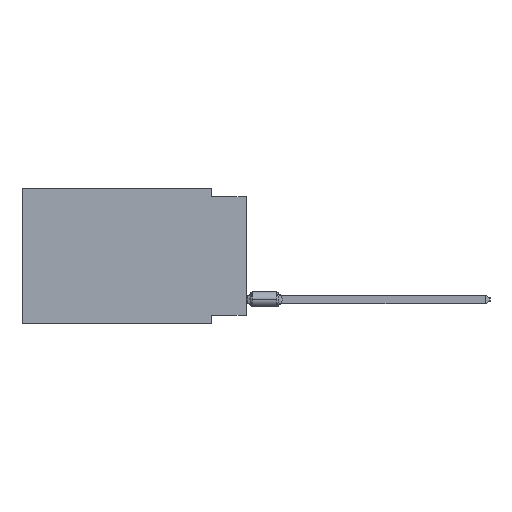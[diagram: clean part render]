
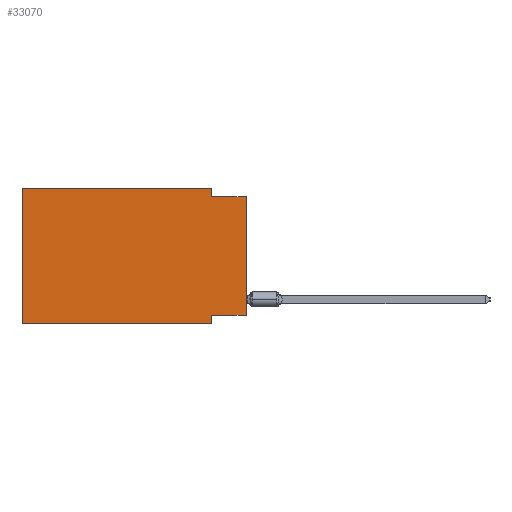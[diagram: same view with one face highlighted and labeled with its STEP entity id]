
A CAD part, left-side view. The second image highlights one B-rep face of the part: STEP entity #33070.
In plain terms, the highlighted planar face has unit normal (-1, 0, 0).
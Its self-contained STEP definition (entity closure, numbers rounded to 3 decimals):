
#898 = VERTEX_POINT ( 'NONE', #55779 ) ;
#2463 = VECTOR ( 'NONE', #65343, 1000. ) ;
#4988 = CARTESIAN_POINT ( 'NONE',  ( 0., 0., -9.271 ) ) ;
#7113 = CARTESIAN_POINT ( 'NONE',  ( 0., 16.383, 0. ) ) ;
#7349 = DIRECTION ( 'NONE',  ( 0., 0., -1. ) ) ;
#8289 = LINE ( 'NONE', #16024, #42178 ) ;
#9789 = VECTOR ( 'NONE', #66621, 1000. ) ;
#11398 = CARTESIAN_POINT ( 'NONE',  ( 0., 16.383, 0. ) ) ;
#13105 = CARTESIAN_POINT ( 'NONE',  ( 0., 0., -0.635 ) ) ;
#13877 = CARTESIAN_POINT ( 'NONE',  ( 0., 16.383, 0. ) ) ;
#13968 = LINE ( 'NONE', #78731, #74807 ) ;
#14330 = DIRECTION ( 'NONE',  ( 0., 1., 0. ) ) ;
#14442 = DIRECTION ( 'NONE',  ( 0., -1., 0. ) ) ;
#16024 = CARTESIAN_POINT ( 'NONE',  ( 0., 0., -9.271 ) ) ;
#18161 = CARTESIAN_POINT ( 'NONE',  ( 0., 0., -0.635 ) ) ;
#18649 = CARTESIAN_POINT ( 'NONE',  ( 0., 2.54, -9.906 ) ) ;
#18819 = EDGE_LOOP ( 'NONE', ( #31350, #49505, #48549, #21379, #64350, #65638, #46109, #35503 ) ) ;
#19003 = DIRECTION ( 'NONE',  ( 1., 0., 0. ) ) ;
#20897 = LINE ( 'NONE', #7113, #51537 ) ;
#21379 = ORIENTED_EDGE ( 'NONE', *, *, #43178, .F. ) ;
#22263 = EDGE_CURVE ( 'NONE', #898, #44504, #66472, .T. ) ;
#25463 = FACE_OUTER_BOUND ( 'NONE', #18819, .T. ) ;
#26371 = EDGE_CURVE ( 'NONE', #33821, #83143, #81209, .T. ) ;
#29829 = DIRECTION ( 'NONE',  ( 0., 0., 1. ) ) ;
#31350 = ORIENTED_EDGE ( 'NONE', *, *, #26371, .T. ) ;
#33070 = ADVANCED_FACE ( 'NONE', ( #25463 ), #58725, .F. ) ;
#33551 = VECTOR ( 'NONE', #66620, 1000. ) ;
#33821 = VERTEX_POINT ( 'NONE', #4988 ) ;
#34724 = AXIS2_PLACEMENT_3D ( 'NONE', #51799, #19003, #45318 ) ;
#35503 = ORIENTED_EDGE ( 'NONE', *, *, #42030, .F. ) ;
#39844 = LINE ( 'NONE', #40260, #33551 ) ;
#40260 = CARTESIAN_POINT ( 'NONE',  ( 0., 16.383, -9.906 ) ) ;
#42030 = EDGE_CURVE ( 'NONE', #33821, #898, #8289, .T. ) ;
#42178 = VECTOR ( 'NONE', #14330, 1000. ) ;
#43178 = EDGE_CURVE ( 'NONE', #59850, #58900, #20897, .T. ) ;
#44185 = LINE ( 'NONE', #11398, #2463 ) ;
#44504 = VERTEX_POINT ( 'NONE', #18649 ) ;
#44828 = CARTESIAN_POINT ( 'NONE',  ( 0., 2.54, 0. ) ) ;
#45318 = DIRECTION ( 'NONE',  ( 0., 0., -1. ) ) ;
#46109 = ORIENTED_EDGE ( 'NONE', *, *, #22263, .F. ) ;
#48549 = ORIENTED_EDGE ( 'NONE', *, *, #66358, .F. ) ;
#49505 = ORIENTED_EDGE ( 'NONE', *, *, #58242, .F. ) ;
#49683 = VERTEX_POINT ( 'NONE', #84803 ) ;
#51537 = VECTOR ( 'NONE', #14442, 1000. ) ;
#51799 = CARTESIAN_POINT ( 'NONE',  ( 0., 16.383, 0. ) ) ;
#53158 = EDGE_CURVE ( 'NONE', #58434, #59850, #44185, .T. ) ;
#54459 = CARTESIAN_POINT ( 'NONE',  ( 0., 0., 0. ) ) ;
#55779 = CARTESIAN_POINT ( 'NONE',  ( 0., 2.54, -9.271 ) ) ;
#58242 = EDGE_CURVE ( 'NONE', #49683, #83143, #59727, .T. ) ;
#58434 = VERTEX_POINT ( 'NONE', #71283 ) ;
#58725 = PLANE ( 'NONE',  #34724 ) ;
#58900 = VERTEX_POINT ( 'NONE', #44828 ) ;
#59727 = LINE ( 'NONE', #13105, #9789 ) ;
#59850 = VERTEX_POINT ( 'NONE', #13877 ) ;
#64350 = ORIENTED_EDGE ( 'NONE', *, *, #53158, .F. ) ;
#65343 = DIRECTION ( 'NONE',  ( 0., 0., 1. ) ) ;
#65638 = ORIENTED_EDGE ( 'NONE', *, *, #69111, .T. ) ;
#66209 = DIRECTION ( 'NONE',  ( 0., 0., -1. ) ) ;
#66358 = EDGE_CURVE ( 'NONE', #58900, #49683, #13968, .T. ) ;
#66472 = LINE ( 'NONE', #77714, #70105 ) ;
#66620 = DIRECTION ( 'NONE',  ( 0., -1., 0. ) ) ;
#66621 = DIRECTION ( 'NONE',  ( 0., -1., 0. ) ) ;
#69111 = EDGE_CURVE ( 'NONE', #58434, #44504, #39844, .T. ) ;
#70105 = VECTOR ( 'NONE', #7349, 1000. ) ;
#71283 = CARTESIAN_POINT ( 'NONE',  ( 0., 16.383, -9.906 ) ) ;
#74807 = VECTOR ( 'NONE', #66209, 1000. ) ;
#77714 = CARTESIAN_POINT ( 'NONE',  ( 0., 2.54, -9.906 ) ) ;
#78093 = VECTOR ( 'NONE', #29829, 1000. ) ;
#78731 = CARTESIAN_POINT ( 'NONE',  ( 0., 2.54, 0. ) ) ;
#81209 = LINE ( 'NONE', #54459, #78093 ) ;
#83143 = VERTEX_POINT ( 'NONE', #18161 ) ;
#84803 = CARTESIAN_POINT ( 'NONE',  ( 0., 2.54, -0.635 ) ) ;
